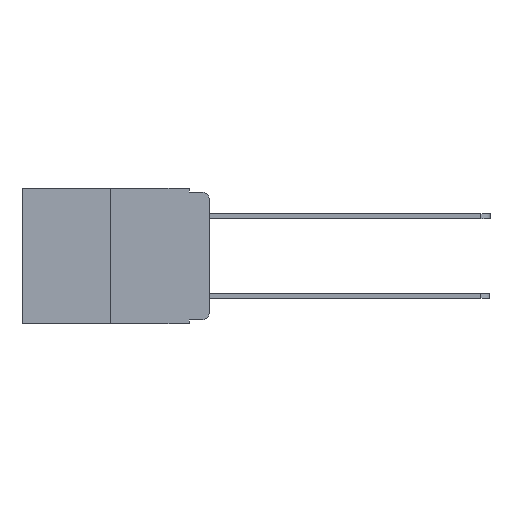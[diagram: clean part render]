
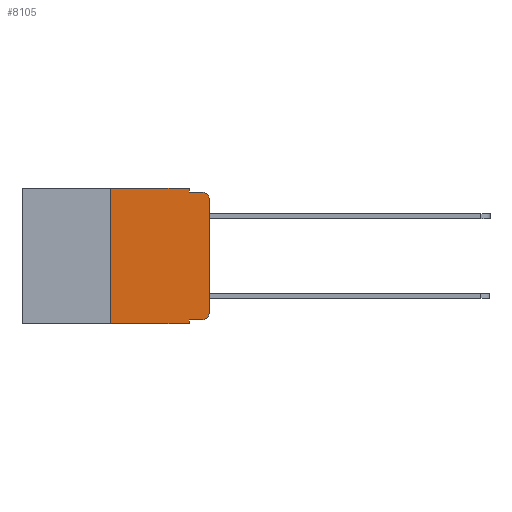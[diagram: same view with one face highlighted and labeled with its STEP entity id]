
A CAD part, left-side view. The second image highlights one B-rep face of the part: STEP entity #8105.
In plain terms, the highlighted planar face has unit normal (-1, 0, 0).
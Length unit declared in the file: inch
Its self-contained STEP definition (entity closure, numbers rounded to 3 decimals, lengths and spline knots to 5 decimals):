
#18 = VERTEX_POINT ( 'NONE', #1753 ) ;
#444 = VERTEX_POINT ( 'NONE', #21138 ) ;
#503 = CARTESIAN_POINT ( 'NONE',  ( 0., 0.051, -0.333 ) ) ;
#556 = LINE ( 'NONE', #13975, #18267 ) ;
#719 = CARTESIAN_POINT ( 'NONE',  ( 0., 0.051, -0.01 ) ) ;
#901 = EDGE_CURVE ( 'NONE', #444, #22152, #556, .T. ) ;
#1322 = CARTESIAN_POINT ( 'NONE',  ( 0., 0.02, -0.01 ) ) ;
#1526 = CARTESIAN_POINT ( 'NONE',  ( 0., 0.25, -0.343 ) ) ;
#1585 = CARTESIAN_POINT ( 'NONE',  ( 0., 0.25, 0. ) ) ;
#1691 = VECTOR ( 'NONE', #4837, 39.37008 ) ;
#1730 = ORIENTED_EDGE ( 'NONE', *, *, #6963, .F. ) ;
#1753 = CARTESIAN_POINT ( 'NONE',  ( 0., 0., -0.313 ) ) ;
#1851 = ORIENTED_EDGE ( 'NONE', *, *, #3778, .F. ) ;
#2102 = CARTESIAN_POINT ( 'NONE',  ( 0., 0.051, -0.333 ) ) ;
#2109 = EDGE_CURVE ( 'NONE', #12220, #14903, #15274, .T. ) ;
#2240 = FACE_OUTER_BOUND ( 'NONE', #2714, .T. ) ;
#2710 = EDGE_CURVE ( 'NONE', #18, #11178, #3075, .T. ) ;
#2714 = EDGE_LOOP ( 'NONE', ( #5793, #6846, #1851, #5019, #3827, #1730, #10984, #9012, #3698, #19356 ) ) ;
#3043 = CARTESIAN_POINT ( 'NONE',  ( 0., 0.051, -0.343 ) ) ;
#3075 = LINE ( 'NONE', #13830, #11985 ) ;
#3366 = VECTOR ( 'NONE', #10626, 39.37008 ) ;
#3698 = ORIENTED_EDGE ( 'NONE', *, *, #5288, .T. ) ;
#3778 = EDGE_CURVE ( 'NONE', #22152, #7964, #4407, .T. ) ;
#3808 = AXIS2_PLACEMENT_3D ( 'NONE', #8828, #20977, #10590 ) ;
#3827 = ORIENTED_EDGE ( 'NONE', *, *, #19560, .F. ) ;
#4130 = CARTESIAN_POINT ( 'NONE',  ( 0., 0.473, 0. ) ) ;
#4302 = CARTESIAN_POINT ( 'NONE',  ( 0., 0.02, -0.313 ) ) ;
#4407 = LINE ( 'NONE', #7942, #9711 ) ;
#4562 = VECTOR ( 'NONE', #7013, 39.37008 ) ;
#4837 = DIRECTION ( 'NONE',  ( 0., -1., 0. ) ) ;
#5019 = ORIENTED_EDGE ( 'NONE', *, *, #901, .F. ) ;
#5288 = EDGE_CURVE ( 'NONE', #5351, #11546, #15130, .T. ) ;
#5351 = VERTEX_POINT ( 'NONE', #503 ) ;
#5759 = VECTOR ( 'NONE', #19664, 39.37008 ) ;
#5793 = ORIENTED_EDGE ( 'NONE', *, *, #2710, .T. ) ;
#6124 = DIRECTION ( 'NONE',  ( 0., 0., -1. ) ) ;
#6575 = AXIS2_PLACEMENT_3D ( 'NONE', #4302, #16635, #6124 ) ;
#6596 = DIRECTION ( 'NONE',  ( -1., 0., 0. ) ) ;
#6846 = ORIENTED_EDGE ( 'NONE', *, *, #14865, .T. ) ;
#6963 = EDGE_CURVE ( 'NONE', #12220, #11697, #20211, .T. ) ;
#7013 = DIRECTION ( 'NONE',  ( 0., 0., 1. ) ) ;
#7193 = CIRCLE ( 'NONE', #16913, 0.02 ) ;
#7757 = DIRECTION ( 'NONE',  ( 0., -1., 0. ) ) ;
#7942 = CARTESIAN_POINT ( 'NONE',  ( 0., 0.051, -0.01 ) ) ;
#7964 = VERTEX_POINT ( 'NONE', #1322 ) ;
#8105 = ADVANCED_FACE ( 'NONE', ( #2240 ), #19279, .F. ) ;
#8828 = CARTESIAN_POINT ( 'NONE',  ( 0., 0.473, 0. ) ) ;
#9012 = ORIENTED_EDGE ( 'NONE', *, *, #18677, .F. ) ;
#9711 = VECTOR ( 'NONE', #20109, 39.37008 ) ;
#10222 = CIRCLE ( 'NONE', #6575, 0.02 ) ;
#10344 = DIRECTION ( 'NONE',  ( 0., 0., 1. ) ) ;
#10552 = CARTESIAN_POINT ( 'NONE',  ( 0., 0.051, 0. ) ) ;
#10590 = DIRECTION ( 'NONE',  ( 0., 0., -1. ) ) ;
#10626 = DIRECTION ( 'NONE',  ( 0., 0., -1. ) ) ;
#10893 = CARTESIAN_POINT ( 'NONE',  ( 0., 0.25, 0. ) ) ;
#10984 = ORIENTED_EDGE ( 'NONE', *, *, #2109, .T. ) ;
#11178 = VERTEX_POINT ( 'NONE', #12931 ) ;
#11222 = EDGE_CURVE ( 'NONE', #11546, #18, #10222, .T. ) ;
#11546 = VERTEX_POINT ( 'NONE', #15814 ) ;
#11697 = VERTEX_POINT ( 'NONE', #10893 ) ;
#11985 = VECTOR ( 'NONE', #10344, 39.37008 ) ;
#12008 = CARTESIAN_POINT ( 'NONE',  ( 0., 0.473, -0.343 ) ) ;
#12220 = VERTEX_POINT ( 'NONE', #1526 ) ;
#12767 = LINE ( 'NONE', #4130, #16845 ) ;
#12806 = LINE ( 'NONE', #10552, #3366 ) ;
#12931 = CARTESIAN_POINT ( 'NONE',  ( 0., 0., -0.03 ) ) ;
#13830 = CARTESIAN_POINT ( 'NONE',  ( 0., 0., 0. ) ) ;
#13975 = CARTESIAN_POINT ( 'NONE',  ( 0., 0.051, 0. ) ) ;
#14865 = EDGE_CURVE ( 'NONE', #11178, #7964, #7193, .T. ) ;
#14903 = VERTEX_POINT ( 'NONE', #3043 ) ;
#15130 = LINE ( 'NONE', #2102, #5759 ) ;
#15274 = LINE ( 'NONE', #12008, #1691 ) ;
#15814 = CARTESIAN_POINT ( 'NONE',  ( 0., 0.02, -0.333 ) ) ;
#16635 = DIRECTION ( 'NONE',  ( -1., 0., 0. ) ) ;
#16845 = VECTOR ( 'NONE', #7757, 39.37008 ) ;
#16913 = AXIS2_PLACEMENT_3D ( 'NONE', #17084, #6596, #18830 ) ;
#17084 = CARTESIAN_POINT ( 'NONE',  ( 0., 0.02, -0.03 ) ) ;
#18267 = VECTOR ( 'NONE', #18491, 39.37008 ) ;
#18491 = DIRECTION ( 'NONE',  ( 0., 0., -1. ) ) ;
#18677 = EDGE_CURVE ( 'NONE', #5351, #14903, #12806, .T. ) ;
#18830 = DIRECTION ( 'NONE',  ( 0., 0., -1. ) ) ;
#19279 = PLANE ( 'NONE',  #3808 ) ;
#19356 = ORIENTED_EDGE ( 'NONE', *, *, #11222, .T. ) ;
#19560 = EDGE_CURVE ( 'NONE', #11697, #444, #12767, .T. ) ;
#19664 = DIRECTION ( 'NONE',  ( 0., -1., 0. ) ) ;
#20109 = DIRECTION ( 'NONE',  ( 0., -1., 0. ) ) ;
#20211 = LINE ( 'NONE', #1585, #4562 ) ;
#20977 = DIRECTION ( 'NONE',  ( 1., 0., 0. ) ) ;
#21138 = CARTESIAN_POINT ( 'NONE',  ( 0., 0.051, 0. ) ) ;
#22152 = VERTEX_POINT ( 'NONE', #719 ) ;
